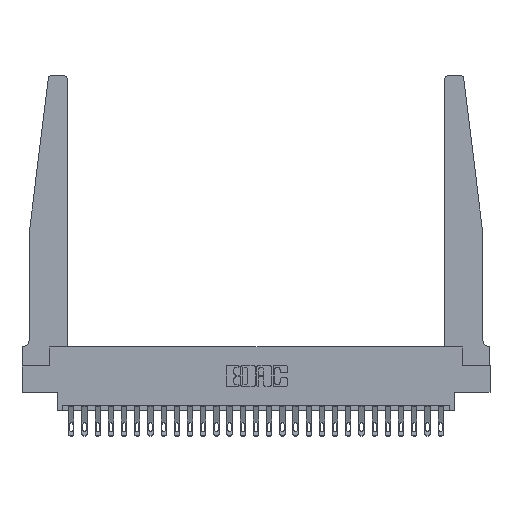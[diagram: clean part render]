
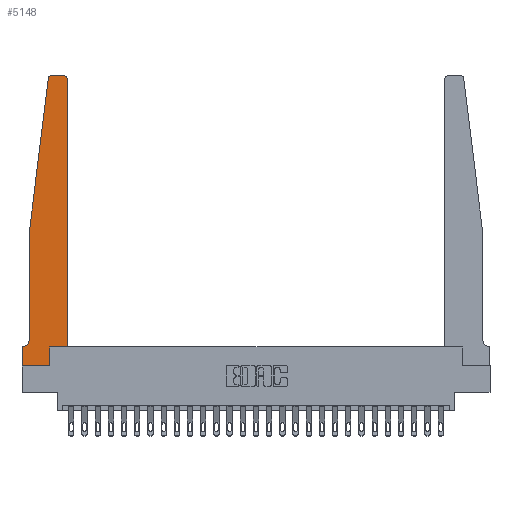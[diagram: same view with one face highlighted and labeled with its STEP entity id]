
A CAD part, top view. The second image highlights one B-rep face of the part: STEP entity #5148.
In plain terms, the highlighted planar face has unit normal (0, 0, 1).
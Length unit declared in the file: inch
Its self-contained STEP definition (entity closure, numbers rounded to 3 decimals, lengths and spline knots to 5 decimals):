
#48 = CARTESIAN_POINT ( 'NONE',  ( 0.065, 0.2375, 0.37 ) ) ;
#373 = CARTESIAN_POINT ( 'NONE',  ( 0.27653, 2.75, 0.37 ) ) ;
#850 = VECTOR ( 'NONE', #13264, 39.37008 ) ;
#1294 = CIRCLE ( 'NONE', #4477, 0.03 ) ;
#1315 = CARTESIAN_POINT ( 'NONE',  ( 0.27653, 2.72, 0.37 ) ) ;
#1501 = CARTESIAN_POINT ( 'NONE',  ( 0.065, 1.25, 0.37 ) ) ;
#1529 = DIRECTION ( 'NONE',  ( 1., 0., 0. ) ) ;
#1626 = ORIENTED_EDGE ( 'NONE', *, *, #20213, .T. ) ;
#1673 = CARTESIAN_POINT ( 'NONE',  ( 0.395, 2.72, 0.37 ) ) ;
#2276 = FACE_OUTER_BOUND ( 'NONE', #8604, .T. ) ;
#2568 = ORIENTED_EDGE ( 'NONE', *, *, #18937, .T. ) ;
#2784 = CARTESIAN_POINT ( 'NONE',  ( 0.425, 2.72, 0.37 ) ) ;
#2959 = ORIENTED_EDGE ( 'NONE', *, *, #13742, .T. ) ;
#3314 = DIRECTION ( 'NONE',  ( 1., 0., 0. ) ) ;
#3501 = DIRECTION ( 'NONE',  ( -0.122, -0.992, 0. ) ) ;
#3669 = DIRECTION ( 'NONE',  ( 1., 0., 0. ) ) ;
#3982 = CARTESIAN_POINT ( 'NONE',  ( 0.425, 0.18, 0.37 ) ) ;
#4188 = VERTEX_POINT ( 'NONE', #9854 ) ;
#4194 = VECTOR ( 'NONE', #3501, 39.37008 ) ;
#4329 = VERTEX_POINT ( 'NONE', #10278 ) ;
#4477 = AXIS2_PLACEMENT_3D ( 'NONE', #1315, #15392, #3314 ) ;
#4485 = ORIENTED_EDGE ( 'NONE', *, *, #24733, .T. ) ;
#4922 = CARTESIAN_POINT ( 'NONE',  ( 0.015, 0.2375, 0.37 ) ) ;
#5147 = VERTEX_POINT ( 'NONE', #2784 ) ;
#5148 = ADVANCED_FACE ( 'NONE', ( #2276 ), #22894, .T. ) ;
#5272 = ORIENTED_EDGE ( 'NONE', *, *, #17883, .T. ) ;
#5511 = CIRCLE ( 'NONE', #21277, 0.05 ) ;
#6631 = VERTEX_POINT ( 'NONE', #7824 ) ;
#6768 = CARTESIAN_POINT ( 'NONE',  ( 0.065, 1.25, 0.37 ) ) ;
#6831 = VERTEX_POINT ( 'NONE', #8427 ) ;
#6891 = DIRECTION ( 'NONE',  ( -1., 0., 0. ) ) ;
#6962 = DIRECTION ( 'NONE',  ( -1., 0., 0. ) ) ;
#7299 = VERTEX_POINT ( 'NONE', #22001 ) ;
#7325 = VERTEX_POINT ( 'NONE', #48 ) ;
#7512 = CARTESIAN_POINT ( 'NONE',  ( 0., 0., 0.37 ) ) ;
#7708 = DIRECTION ( 'NONE',  ( 0., 1., 0. ) ) ;
#7824 = CARTESIAN_POINT ( 'NONE',  ( 0.2605, 0.18, 0.37 ) ) ;
#7875 = EDGE_CURVE ( 'NONE', #6631, #14457, #10407, .T. ) ;
#8218 = VECTOR ( 'NONE', #7708, 39.37008 ) ;
#8239 = VECTOR ( 'NONE', #25436, 39.37008 ) ;
#8264 = VECTOR ( 'NONE', #6891, 39.37008 ) ;
#8427 = CARTESIAN_POINT ( 'NONE',  ( 0.2605, 0., 0.37 ) ) ;
#8604 = EDGE_LOOP ( 'NONE', ( #14462, #12516, #2959, #2568, #4485, #5272, #19681, #12810, #1626, #21817, #11360, #16481 ) ) ;
#8756 = VERTEX_POINT ( 'NONE', #20081 ) ;
#9085 = LINE ( 'NONE', #20474, #24397 ) ;
#9449 = CARTESIAN_POINT ( 'NONE',  ( 0.2605, 0.18, 0.37 ) ) ;
#9854 = CARTESIAN_POINT ( 'NONE',  ( 0.24675, 2.72367, 0.37 ) ) ;
#10278 = CARTESIAN_POINT ( 'NONE',  ( 0., 0., 0.37 ) ) ;
#10389 = DIRECTION ( 'NONE',  ( 1., 0., 0. ) ) ;
#10407 = LINE ( 'NONE', #19520, #15158 ) ;
#10671 = LINE ( 'NONE', #7512, #20702 ) ;
#10891 = DIRECTION ( 'NONE',  ( 0., 0., 1. ) ) ;
#11235 = CARTESIAN_POINT ( 'NONE',  ( 0.065, 1.25, 0.37 ) ) ;
#11360 = ORIENTED_EDGE ( 'NONE', *, *, #16360, .T. ) ;
#12258 = VECTOR ( 'NONE', #24098, 39.37008 ) ;
#12516 = ORIENTED_EDGE ( 'NONE', *, *, #16696, .T. ) ;
#12810 = ORIENTED_EDGE ( 'NONE', *, *, #22960, .T. ) ;
#12895 = LINE ( 'NONE', #22132, #12258 ) ;
#13264 = DIRECTION ( 'NONE',  ( 0., -1., 0. ) ) ;
#13312 = VERTEX_POINT ( 'NONE', #15686 ) ;
#13652 = LINE ( 'NONE', #16915, #8264 ) ;
#13742 = EDGE_CURVE ( 'NONE', #4188, #25715, #14949, .T. ) ;
#13777 = EDGE_CURVE ( 'NONE', #5147, #7299, #19013, .T. ) ;
#14457 = VERTEX_POINT ( 'NONE', #3982 ) ;
#14462 = ORIENTED_EDGE ( 'NONE', *, *, #14759, .T. ) ;
#14759 = EDGE_CURVE ( 'NONE', #7299, #20632, #13652, .T. ) ;
#14861 = CARTESIAN_POINT ( 'NONE',  ( 0., 0.1875, 0.37 ) ) ;
#14949 = LINE ( 'NONE', #1501, #4194 ) ;
#15158 = VECTOR ( 'NONE', #1529, 39.37008 ) ;
#15392 = DIRECTION ( 'NONE',  ( 0., 0., 1. ) ) ;
#15686 = CARTESIAN_POINT ( 'NONE',  ( 0., 0.1875, 0.37 ) ) ;
#15735 = DIRECTION ( 'NONE',  ( 0., 0., 1. ) ) ;
#16360 = EDGE_CURVE ( 'NONE', #14457, #5147, #18276, .T. ) ;
#16481 = ORIENTED_EDGE ( 'NONE', *, *, #13777, .T. ) ;
#16696 = EDGE_CURVE ( 'NONE', #20632, #4188, #1294, .T. ) ;
#16903 = LINE ( 'NONE', #11235, #850 ) ;
#16915 = CARTESIAN_POINT ( 'NONE',  ( 0.25, 2.75, 0.37 ) ) ;
#17614 = DIRECTION ( 'NONE',  ( 0., -1., 0. ) ) ;
#17718 = CARTESIAN_POINT ( 'NONE',  ( 0.425, 0.18, 0.37 ) ) ;
#17883 = EDGE_CURVE ( 'NONE', #8756, #13312, #12895, .T. ) ;
#18276 = LINE ( 'NONE', #17718, #8218 ) ;
#18937 = EDGE_CURVE ( 'NONE', #25715, #7325, #16903, .T. ) ;
#19007 = DIRECTION ( 'NONE',  ( 0., 0., -1. ) ) ;
#19013 = CIRCLE ( 'NONE', #19763, 0.03 ) ;
#19520 = CARTESIAN_POINT ( 'NONE',  ( 0.425, 0.18, 0.37 ) ) ;
#19681 = ORIENTED_EDGE ( 'NONE', *, *, #22637, .T. ) ;
#19763 = AXIS2_PLACEMENT_3D ( 'NONE', #1673, #15735, #3669 ) ;
#20081 = CARTESIAN_POINT ( 'NONE',  ( 0.015, 0.1875, 0.37 ) ) ;
#20213 = EDGE_CURVE ( 'NONE', #6831, #6631, #24197, .T. ) ;
#20474 = CARTESIAN_POINT ( 'NONE',  ( 0., 0., 0.37 ) ) ;
#20632 = VERTEX_POINT ( 'NONE', #373 ) ;
#20702 = VECTOR ( 'NONE', #17614, 39.37008 ) ;
#20834 = AXIS2_PLACEMENT_3D ( 'NONE', #14861, #10891, #24840 ) ;
#21277 = AXIS2_PLACEMENT_3D ( 'NONE', #4922, #19007, #6962 ) ;
#21817 = ORIENTED_EDGE ( 'NONE', *, *, #7875, .T. ) ;
#22001 = CARTESIAN_POINT ( 'NONE',  ( 0.395, 2.75, 0.37 ) ) ;
#22132 = CARTESIAN_POINT ( 'NONE',  ( 0.065, 0.1875, 0.37 ) ) ;
#22637 = EDGE_CURVE ( 'NONE', #13312, #4329, #10671, .T. ) ;
#22894 = PLANE ( 'NONE',  #20834 ) ;
#22960 = EDGE_CURVE ( 'NONE', #4329, #6831, #9085, .T. ) ;
#24098 = DIRECTION ( 'NONE',  ( -1., 0., 0. ) ) ;
#24197 = LINE ( 'NONE', #9449, #8239 ) ;
#24397 = VECTOR ( 'NONE', #10389, 39.37008 ) ;
#24733 = EDGE_CURVE ( 'NONE', #7325, #8756, #5511, .T. ) ;
#24840 = DIRECTION ( 'NONE',  ( 1., 0., 0. ) ) ;
#25436 = DIRECTION ( 'NONE',  ( 0., 1., 0. ) ) ;
#25715 = VERTEX_POINT ( 'NONE', #6768 ) ;
